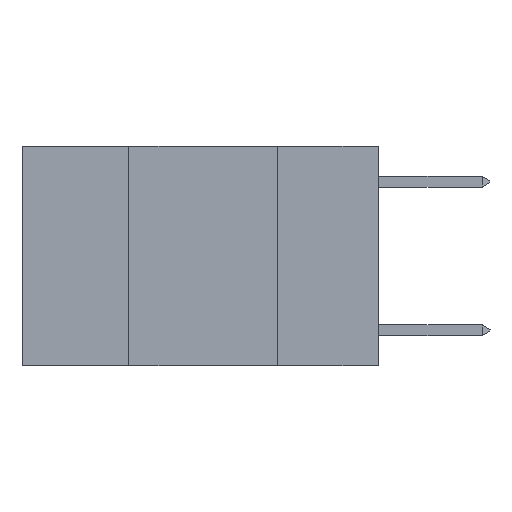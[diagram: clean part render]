
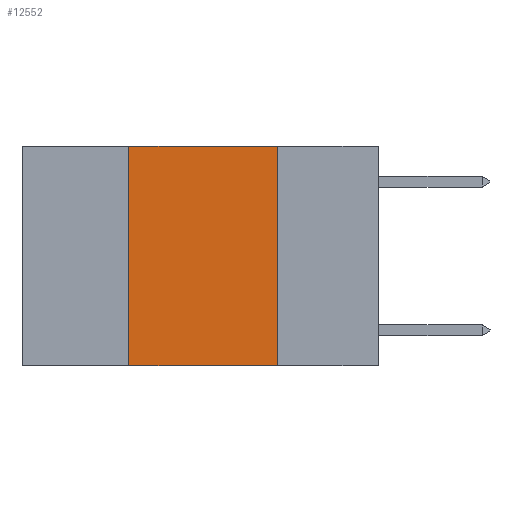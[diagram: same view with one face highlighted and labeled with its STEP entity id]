
A CAD part, left-side view. The second image highlights one B-rep face of the part: STEP entity #12552.
In plain terms, the highlighted planar face has unit normal (-1, 0, 0).
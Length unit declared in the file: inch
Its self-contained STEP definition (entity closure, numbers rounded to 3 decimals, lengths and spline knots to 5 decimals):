
#1518 = FACE_OUTER_BOUND ( 'NONE', #18418, .T. ) ;
#1528 = VECTOR ( 'NONE', #6801, 39.37008 ) ;
#1701 = LINE ( 'NONE', #5868, #1528 ) ;
#3469 = DIRECTION ( 'NONE',  ( 0., 0., -1. ) ) ;
#3494 = DIRECTION ( 'NONE',  ( 1., 0., 0. ) ) ;
#3499 = CARTESIAN_POINT ( 'NONE',  ( 0., 0.6, 0. ) ) ;
#3662 = ORIENTED_EDGE ( 'NONE', *, *, #9527, .F. ) ;
#3800 = VERTEX_POINT ( 'NONE', #6151 ) ;
#4240 = ORIENTED_EDGE ( 'NONE', *, *, #24878, .F. ) ;
#4502 = ORIENTED_EDGE ( 'NONE', *, *, #6577, .T. ) ;
#5112 = VECTOR ( 'NONE', #15126, 39.37008 ) ;
#5239 = LINE ( 'NONE', #15182, #5112 ) ;
#5868 = CARTESIAN_POINT ( 'NONE',  ( 0., 0.17, 0. ) ) ;
#6005 = ORIENTED_EDGE ( 'NONE', *, *, #9896, .F. ) ;
#6151 = CARTESIAN_POINT ( 'NONE',  ( 0., 0.17, 0. ) ) ;
#6577 = EDGE_CURVE ( 'NONE', #20793, #9267, #14576, .T. ) ;
#6801 = DIRECTION ( 'NONE',  ( 0., 0., -1. ) ) ;
#7158 = VECTOR ( 'NONE', #9455, 39.37008 ) ;
#7212 = LINE ( 'NONE', #7393, #7158 ) ;
#7393 = CARTESIAN_POINT ( 'NONE',  ( 0., 0.42, 0. ) ) ;
#8807 = VERTEX_POINT ( 'NONE', #22845 ) ;
#8932 = CARTESIAN_POINT ( 'NONE',  ( 0., 0.6, -0.37 ) ) ;
#9267 = VERTEX_POINT ( 'NONE', #21347 ) ;
#9455 = DIRECTION ( 'NONE',  ( 0., 0., 1. ) ) ;
#9527 = EDGE_CURVE ( 'NONE', #8807, #3800, #5239, .T. ) ;
#9896 = EDGE_CURVE ( 'NONE', #3800, #9267, #1701, .T. ) ;
#9937 = DIRECTION ( 'NONE',  ( 0., -1., 0. ) ) ;
#12552 = ADVANCED_FACE ( 'NONE', ( #1518 ), #18129, .F. ) ;
#13970 = VECTOR ( 'NONE', #9937, 39.37008 ) ;
#14576 = LINE ( 'NONE', #8932, #13970 ) ;
#14679 = AXIS2_PLACEMENT_3D ( 'NONE', #3499, #3494, #3469 ) ;
#15126 = DIRECTION ( 'NONE',  ( 0., -1., 0. ) ) ;
#15182 = CARTESIAN_POINT ( 'NONE',  ( 0., 0.6, 0. ) ) ;
#18129 = PLANE ( 'NONE',  #14679 ) ;
#18418 = EDGE_LOOP ( 'NONE', ( #6005, #3662, #4240, #4502 ) ) ;
#20793 = VERTEX_POINT ( 'NONE', #20796 ) ;
#20796 = CARTESIAN_POINT ( 'NONE',  ( 0., 0.42, -0.37 ) ) ;
#21347 = CARTESIAN_POINT ( 'NONE',  ( 0., 0.17, -0.37 ) ) ;
#22845 = CARTESIAN_POINT ( 'NONE',  ( 0., 0.42, 0. ) ) ;
#24878 = EDGE_CURVE ( 'NONE', #20793, #8807, #7212, .T. ) ;
